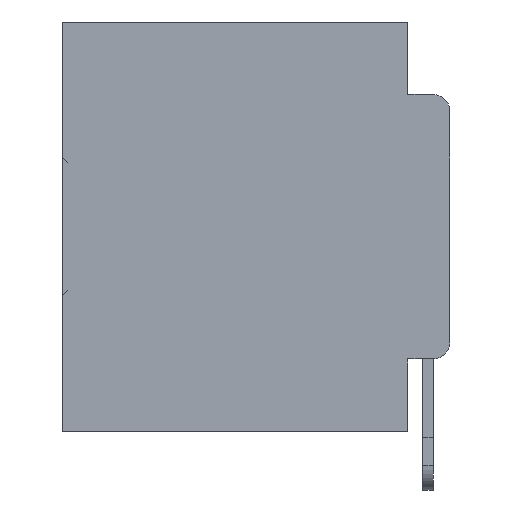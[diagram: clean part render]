
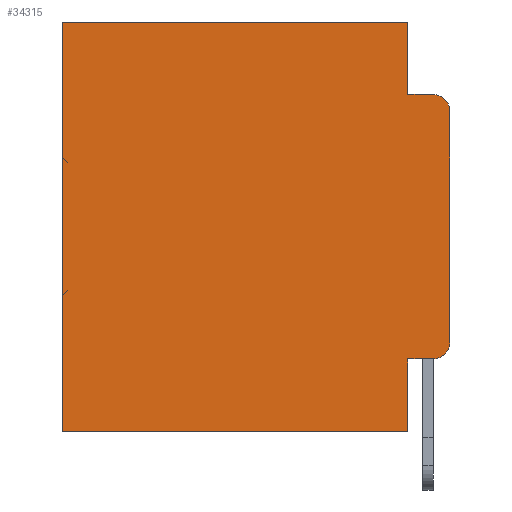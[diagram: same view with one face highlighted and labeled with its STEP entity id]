
A CAD part, left-side view. The second image highlights one B-rep face of the part: STEP entity #34315.
In plain terms, the highlighted planar face has unit normal (-1, 0, 0).
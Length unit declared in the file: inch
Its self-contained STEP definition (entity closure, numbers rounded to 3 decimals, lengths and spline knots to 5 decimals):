
#127 = VECTOR ( 'NONE', #28259, 39.37008 ) ;
#1058 = VECTOR ( 'NONE', #14551, 39.37008 ) ;
#2039 = CARTESIAN_POINT ( 'NONE',  ( 0.298, 0.051, -0.4115 ) ) ;
#2104 = CARTESIAN_POINT ( 'NONE',  ( 0.298, 0.02, -0.0885 ) ) ;
#2263 = VERTEX_POINT ( 'NONE', #2104 ) ;
#3204 = ORIENTED_EDGE ( 'NONE', *, *, #10599, .F. ) ;
#3463 = DIRECTION ( 'NONE',  ( -1., 0., 0. ) ) ;
#5136 = ORIENTED_EDGE ( 'NONE', *, *, #33689, .T. ) ;
#5977 = VERTEX_POINT ( 'NONE', #23552 ) ;
#6931 = DIRECTION ( 'NONE',  ( 0., 1., 0. ) ) ;
#7160 = VERTEX_POINT ( 'NONE', #34212 ) ;
#7478 = LINE ( 'NONE', #10458, #22379 ) ;
#7941 = LINE ( 'NONE', #9086, #127 ) ;
#8776 = VERTEX_POINT ( 'NONE', #23487 ) ;
#9086 = CARTESIAN_POINT ( 'NONE',  ( 0.298, 0.051, -0.0885 ) ) ;
#9396 = VECTOR ( 'NONE', #20988, 39.37008 ) ;
#9453 = AXIS2_PLACEMENT_3D ( 'NONE', #20472, #3463, #23139 ) ;
#9629 = EDGE_CURVE ( 'NONE', #8776, #2263, #7941, .T. ) ;
#10375 = VERTEX_POINT ( 'NONE', #14758 ) ;
#10458 = CARTESIAN_POINT ( 'NONE',  ( 0.298, 0.051, 0. ) ) ;
#10599 = EDGE_CURVE ( 'NONE', #12707, #32377, #7478, .T. ) ;
#11168 = EDGE_CURVE ( 'NONE', #24537, #7160, #18090, .T. ) ;
#11676 = CARTESIAN_POINT ( 'NONE',  ( 0.298, 0., -0.5 ) ) ;
#11917 = ORIENTED_EDGE ( 'NONE', *, *, #18849, .T. ) ;
#11999 = CARTESIAN_POINT ( 'NONE',  ( 0.298, 0.02, -0.3915 ) ) ;
#12496 = EDGE_CURVE ( 'NONE', #32377, #5977, #23613, .T. ) ;
#12707 = VERTEX_POINT ( 'NONE', #23497 ) ;
#12827 = ORIENTED_EDGE ( 'NONE', *, *, #14264, .F. ) ;
#13321 = FACE_OUTER_BOUND ( 'NONE', #14205, .T. ) ;
#14205 = EDGE_LOOP ( 'NONE', ( #25976, #21457, #24683, #12827, #28865, #21844, #34206, #3204, #11917, #5136 ) ) ;
#14264 = EDGE_CURVE ( 'NONE', #10375, #8776, #32168, .T. ) ;
#14499 = VERTEX_POINT ( 'NONE', #17253 ) ;
#14551 = DIRECTION ( 'NONE',  ( 0., 1., 0. ) ) ;
#14758 = CARTESIAN_POINT ( 'NONE',  ( 0.298, 0.051, 0. ) ) ;
#14875 = DIRECTION ( 'NONE',  ( 0., 0., -1. ) ) ;
#15845 = VECTOR ( 'NONE', #6931, 39.37008 ) ;
#15907 = CARTESIAN_POINT ( 'NONE',  ( 0.298, 0., 0. ) ) ;
#16952 = VECTOR ( 'NONE', #34514, 39.37008 ) ;
#17000 = LINE ( 'NONE', #26171, #9396 ) ;
#17234 = DIRECTION ( 'NONE',  ( 0., 0., -1. ) ) ;
#17253 = CARTESIAN_POINT ( 'NONE',  ( 0.298, 0.02, -0.4115 ) ) ;
#18090 = LINE ( 'NONE', #15907, #16952 ) ;
#18740 = CARTESIAN_POINT ( 'NONE',  ( 0.298, 0., -0.1085 ) ) ;
#18849 = EDGE_CURVE ( 'NONE', #12707, #14499, #29371, .T. ) ;
#20057 = AXIS2_PLACEMENT_3D ( 'NONE', #30500, #33144, #17234 ) ;
#20472 = CARTESIAN_POINT ( 'NONE',  ( 0.298, 0.02, -0.1085 ) ) ;
#20988 = DIRECTION ( 'NONE',  ( 0., 0., -1. ) ) ;
#21457 = ORIENTED_EDGE ( 'NONE', *, *, #33730, .T. ) ;
#21844 = ORIENTED_EDGE ( 'NONE', *, *, #29293, .T. ) ;
#22379 = VECTOR ( 'NONE', #34784, 39.37008 ) ;
#23139 = DIRECTION ( 'NONE',  ( 0., 0., -1. ) ) ;
#23487 = CARTESIAN_POINT ( 'NONE',  ( 0.298, 0.051, -0.0885 ) ) ;
#23497 = CARTESIAN_POINT ( 'NONE',  ( 0.298, 0.051, -0.4115 ) ) ;
#23552 = CARTESIAN_POINT ( 'NONE',  ( 0.298, 0.473, -0.5 ) ) ;
#23613 = LINE ( 'NONE', #11676, #1058 ) ;
#23646 = CARTESIAN_POINT ( 'NONE',  ( 0.298, 0., 0. ) ) ;
#24537 = VERTEX_POINT ( 'NONE', #18740 ) ;
#24683 = ORIENTED_EDGE ( 'NONE', *, *, #9629, .F. ) ;
#24772 = CIRCLE ( 'NONE', #9453, 0.02 ) ;
#25591 = CIRCLE ( 'NONE', #33763, 0.02 ) ;
#25976 = ORIENTED_EDGE ( 'NONE', *, *, #11168, .F. ) ;
#26171 = CARTESIAN_POINT ( 'NONE',  ( 0.298, 0.473, 0. ) ) ;
#27067 = CARTESIAN_POINT ( 'NONE',  ( 0.298, 0.051, 0. ) ) ;
#27329 = CARTESIAN_POINT ( 'NONE',  ( 0.298, 0.051, -0.5 ) ) ;
#27338 = EDGE_CURVE ( 'NONE', #10375, #28900, #30044, .T. ) ;
#27835 = PLANE ( 'NONE',  #20057 ) ;
#28259 = DIRECTION ( 'NONE',  ( 0., -1., 0. ) ) ;
#28865 = ORIENTED_EDGE ( 'NONE', *, *, #27338, .T. ) ;
#28900 = VERTEX_POINT ( 'NONE', #29663 ) ;
#29293 = EDGE_CURVE ( 'NONE', #28900, #5977, #17000, .T. ) ;
#29371 = LINE ( 'NONE', #2039, #35545 ) ;
#29663 = CARTESIAN_POINT ( 'NONE',  ( 0.298, 0.473, 0. ) ) ;
#29712 = DIRECTION ( 'NONE',  ( 0., 0., -1. ) ) ;
#30044 = LINE ( 'NONE', #23646, #15845 ) ;
#30500 = CARTESIAN_POINT ( 'NONE',  ( 0.298, 0., 0. ) ) ;
#30897 = DIRECTION ( 'NONE',  ( -1., 0., 0. ) ) ;
#32168 = LINE ( 'NONE', #27067, #32976 ) ;
#32377 = VERTEX_POINT ( 'NONE', #27329 ) ;
#32976 = VECTOR ( 'NONE', #29712, 39.37008 ) ;
#33144 = DIRECTION ( 'NONE',  ( 1., 0., 0. ) ) ;
#33689 = EDGE_CURVE ( 'NONE', #14499, #7160, #25591, .T. ) ;
#33730 = EDGE_CURVE ( 'NONE', #24537, #2263, #24772, .T. ) ;
#33763 = AXIS2_PLACEMENT_3D ( 'NONE', #11999, #30897, #14875 ) ;
#34206 = ORIENTED_EDGE ( 'NONE', *, *, #12496, .F. ) ;
#34212 = CARTESIAN_POINT ( 'NONE',  ( 0.298, 0., -0.3915 ) ) ;
#34315 = ADVANCED_FACE ( 'NONE', ( #13321 ), #27835, .F. ) ;
#34514 = DIRECTION ( 'NONE',  ( 0., 0., -1. ) ) ;
#34784 = DIRECTION ( 'NONE',  ( 0., 0., -1. ) ) ;
#35112 = DIRECTION ( 'NONE',  ( 0., -1., 0. ) ) ;
#35545 = VECTOR ( 'NONE', #35112, 39.37008 ) ;
